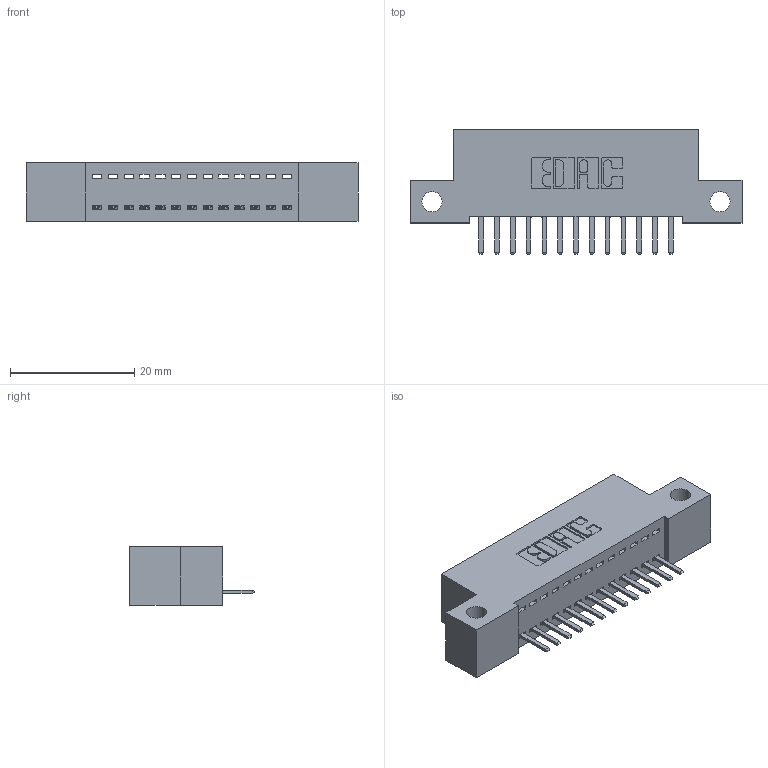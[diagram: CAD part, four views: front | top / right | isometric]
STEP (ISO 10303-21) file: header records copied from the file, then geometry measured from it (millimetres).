
FILE_DESCRIPTION (( 'STEP AP203' ), '1' );
FILE_NAME ('392-013-520-112.STEP', '2019-10-07T01:48:00', ( '' ), ( '' ), 'SwSTEP 2.0', 'SolidWorks 2016', '' );
FILE_SCHEMA (( 'CONFIG_CONTROL_DESIGN' ));
Length unit declared in the file: inch
Products named in the file (3): 345-292-001_345-293-120; 392-013-520-112; 342 Part_Side Mount
Assembly tree (14 placements, depth 2):
  392-013-520-112
    342 Part_Side Mount
    345-292-001_345-293-120  x13
Bounding box: 53.34 x 20.02 x 9.4 mm (x, y, z)
Volume: 4458.7 mm3; surface area: 5723.3 mm2
Topology: 14 solids, 14 shells, 916 faces, 2691 edges, 1758 vertices
Faces by surface type: plane 638, cylinder 278
Entity records: 11683 total; most frequent: CARTESIAN_POINT 2037, ORIENTED_EDGE 1974, DIRECTION 1765, EDGE_CURVE 987, VECTOR 855, LINE 855, VERTEX_POINT 654, AXIS2_PLACEMENT_3D 455
